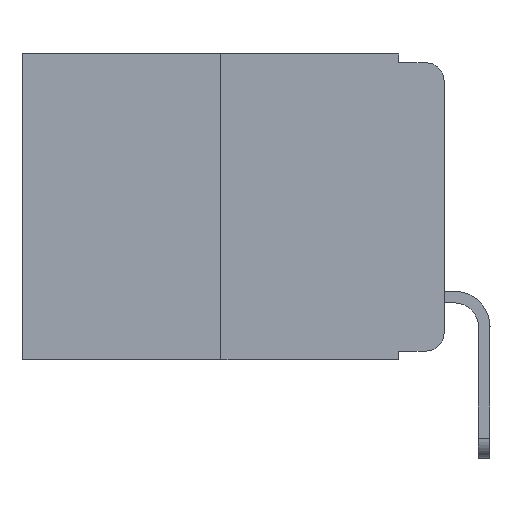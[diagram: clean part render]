
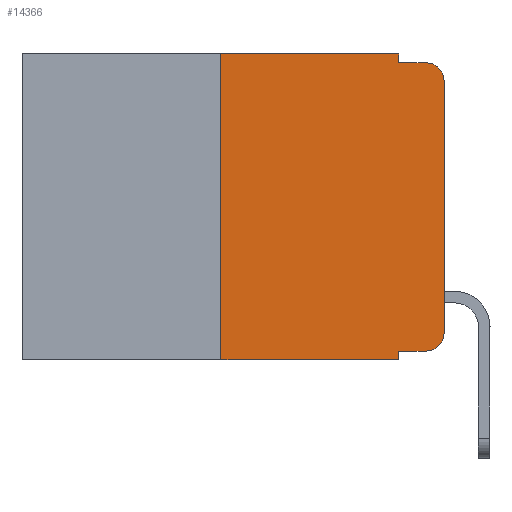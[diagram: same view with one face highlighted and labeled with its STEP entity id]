
A CAD part, left-side view. The second image highlights one B-rep face of the part: STEP entity #14366.
In plain terms, the highlighted planar face has unit normal (-1, 0, 0).
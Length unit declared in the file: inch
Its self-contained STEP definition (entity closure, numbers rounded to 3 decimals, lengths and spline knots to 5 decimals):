
#101 = ORIENTED_EDGE ( 'NONE', *, *, #12572, .F. ) ;
#432 = LINE ( 'NONE', #2818, #16516 ) ;
#800 = ORIENTED_EDGE ( 'NONE', *, *, #5984, .F. ) ;
#1162 = DIRECTION ( 'NONE',  ( 0., -1., 0. ) ) ;
#1563 = VERTEX_POINT ( 'NONE', #6988 ) ;
#1771 = PLANE ( 'NONE',  #7814 ) ;
#2067 = CARTESIAN_POINT ( 'NONE',  ( 0., 0.051, -0.333 ) ) ;
#2547 = CARTESIAN_POINT ( 'NONE',  ( 0., 0.051, 0. ) ) ;
#2598 = EDGE_CURVE ( 'NONE', #6608, #16925, #14028, .T. ) ;
#2611 = LINE ( 'NONE', #17417, #6875 ) ;
#2661 = DIRECTION ( 'NONE',  ( 0., 0., 1. ) ) ;
#2818 = CARTESIAN_POINT ( 'NONE',  ( 0., 0.051, -0.01 ) ) ;
#2971 = EDGE_CURVE ( 'NONE', #16925, #8553, #14654, .T. ) ;
#3222 = EDGE_CURVE ( 'NONE', #3564, #11962, #9831, .T. ) ;
#3291 = EDGE_CURVE ( 'NONE', #6608, #10903, #9428, .T. ) ;
#3480 = DIRECTION ( 'NONE',  ( 0., -1., 0. ) ) ;
#3562 = CARTESIAN_POINT ( 'NONE',  ( 0., 0.051, -0.333 ) ) ;
#3564 = VERTEX_POINT ( 'NONE', #13071 ) ;
#3582 = LINE ( 'NONE', #16784, #6994 ) ;
#3803 = DIRECTION ( 'NONE',  ( 0., 0., -1. ) ) ;
#4001 = LINE ( 'NONE', #14804, #4896 ) ;
#4154 = CARTESIAN_POINT ( 'NONE',  ( 0., 0.25, -0.343 ) ) ;
#4896 = VECTOR ( 'NONE', #2661, 39.37008 ) ;
#5280 = ORIENTED_EDGE ( 'NONE', *, *, #6143, .T. ) ;
#5527 = VECTOR ( 'NONE', #3480, 39.37008 ) ;
#5622 = DIRECTION ( 'NONE',  ( 0., 0., -1. ) ) ;
#5774 = ORIENTED_EDGE ( 'NONE', *, *, #3222, .T. ) ;
#5799 = CARTESIAN_POINT ( 'NONE',  ( 0., 0.051, 0. ) ) ;
#5824 = EDGE_CURVE ( 'NONE', #12681, #10903, #2611, .T. ) ;
#5893 = VECTOR ( 'NONE', #6876, 39.37008 ) ;
#5984 = EDGE_CURVE ( 'NONE', #1563, #6095, #7042, .T. ) ;
#6095 = VERTEX_POINT ( 'NONE', #7569 ) ;
#6143 = EDGE_CURVE ( 'NONE', #8553, #3564, #3582, .T. ) ;
#6608 = VERTEX_POINT ( 'NONE', #3562 ) ;
#6875 = VECTOR ( 'NONE', #14930, 39.37008 ) ;
#6876 = DIRECTION ( 'NONE',  ( 0., 0., -1. ) ) ;
#6886 = DIRECTION ( 'NONE',  ( 0., -1., 0. ) ) ;
#6988 = CARTESIAN_POINT ( 'NONE',  ( 0., 0.051, 0. ) ) ;
#6992 = AXIS2_PLACEMENT_3D ( 'NONE', #12334, #8073, #15490 ) ;
#6994 = VECTOR ( 'NONE', #8966, 39.37008 ) ;
#7033 = AXIS2_PLACEMENT_3D ( 'NONE', #10697, #16109, #3803 ) ;
#7042 = LINE ( 'NONE', #5799, #7341 ) ;
#7341 = VECTOR ( 'NONE', #5622, 39.37008 ) ;
#7569 = CARTESIAN_POINT ( 'NONE',  ( 0., 0.051, -0.01 ) ) ;
#7814 = AXIS2_PLACEMENT_3D ( 'NONE', #13599, #9346, #14598 ) ;
#7928 = ORIENTED_EDGE ( 'NONE', *, *, #3291, .F. ) ;
#8073 = DIRECTION ( 'NONE',  ( -1., 0., 0. ) ) ;
#8498 = FACE_OUTER_BOUND ( 'NONE', #10156, .T. ) ;
#8553 = VERTEX_POINT ( 'NONE', #11142 ) ;
#8966 = DIRECTION ( 'NONE',  ( 0., 0., 1. ) ) ;
#9346 = DIRECTION ( 'NONE',  ( 1., 0., 0. ) ) ;
#9428 = LINE ( 'NONE', #2547, #5893 ) ;
#9684 = VERTEX_POINT ( 'NONE', #16946 ) ;
#9713 = ORIENTED_EDGE ( 'NONE', *, *, #11466, .F. ) ;
#9831 = CIRCLE ( 'NONE', #7033, 0.02 ) ;
#10156 = EDGE_LOOP ( 'NONE', ( #5280, #5774, #9713, #800, #101, #12143, #13899, #7928, #13300, #14003 ) ) ;
#10540 = CARTESIAN_POINT ( 'NONE',  ( 0., 0.473, 0. ) ) ;
#10697 = CARTESIAN_POINT ( 'NONE',  ( 0., 0.02, -0.03 ) ) ;
#10903 = VERTEX_POINT ( 'NONE', #12150 ) ;
#10975 = EDGE_CURVE ( 'NONE', #12681, #9684, #4001, .T. ) ;
#11142 = CARTESIAN_POINT ( 'NONE',  ( 0., 0., -0.313 ) ) ;
#11386 = CARTESIAN_POINT ( 'NONE',  ( 0., 0.02, -0.01 ) ) ;
#11466 = EDGE_CURVE ( 'NONE', #6095, #11962, #432, .T. ) ;
#11962 = VERTEX_POINT ( 'NONE', #11386 ) ;
#12143 = ORIENTED_EDGE ( 'NONE', *, *, #10975, .F. ) ;
#12150 = CARTESIAN_POINT ( 'NONE',  ( 0., 0.051, -0.343 ) ) ;
#12334 = CARTESIAN_POINT ( 'NONE',  ( 0., 0.02, -0.313 ) ) ;
#12395 = CARTESIAN_POINT ( 'NONE',  ( 0., 0.02, -0.333 ) ) ;
#12572 = EDGE_CURVE ( 'NONE', #9684, #1563, #16123, .T. ) ;
#12681 = VERTEX_POINT ( 'NONE', #4154 ) ;
#13071 = CARTESIAN_POINT ( 'NONE',  ( 0., 0., -0.03 ) ) ;
#13300 = ORIENTED_EDGE ( 'NONE', *, *, #2598, .T. ) ;
#13599 = CARTESIAN_POINT ( 'NONE',  ( 0., 0.473, 0. ) ) ;
#13899 = ORIENTED_EDGE ( 'NONE', *, *, #5824, .T. ) ;
#14003 = ORIENTED_EDGE ( 'NONE', *, *, #2971, .T. ) ;
#14028 = LINE ( 'NONE', #2067, #5527 ) ;
#14366 = ADVANCED_FACE ( 'NONE', ( #8498 ), #1771, .F. ) ;
#14598 = DIRECTION ( 'NONE',  ( 0., 0., -1. ) ) ;
#14654 = CIRCLE ( 'NONE', #6992, 0.02 ) ;
#14804 = CARTESIAN_POINT ( 'NONE',  ( 0., 0.25, 0. ) ) ;
#14930 = DIRECTION ( 'NONE',  ( 0., -1., 0. ) ) ;
#15110 = VECTOR ( 'NONE', #1162, 39.37008 ) ;
#15490 = DIRECTION ( 'NONE',  ( 0., 0., -1. ) ) ;
#16109 = DIRECTION ( 'NONE',  ( -1., 0., 0. ) ) ;
#16123 = LINE ( 'NONE', #10540, #15110 ) ;
#16516 = VECTOR ( 'NONE', #6886, 39.37008 ) ;
#16784 = CARTESIAN_POINT ( 'NONE',  ( 0., 0., 0. ) ) ;
#16925 = VERTEX_POINT ( 'NONE', #12395 ) ;
#16946 = CARTESIAN_POINT ( 'NONE',  ( 0., 0.25, 0. ) ) ;
#17417 = CARTESIAN_POINT ( 'NONE',  ( 0., 0.473, -0.343 ) ) ;
